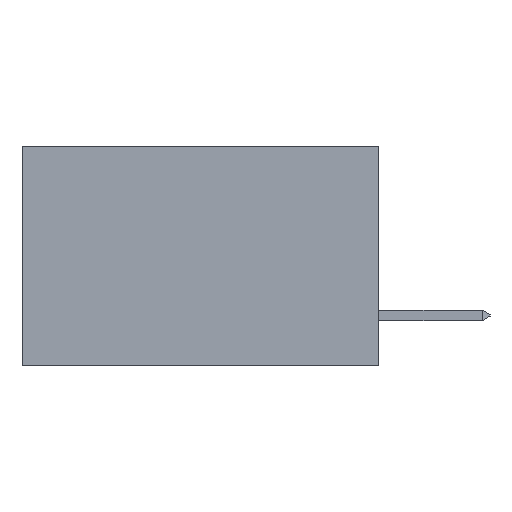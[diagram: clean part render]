
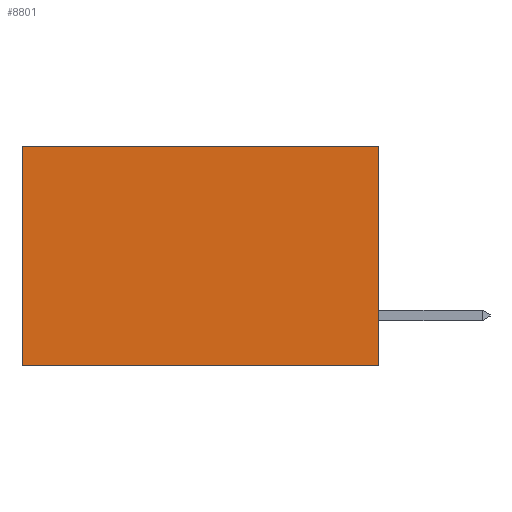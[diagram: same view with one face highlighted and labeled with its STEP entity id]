
A CAD part, left-side view. The second image highlights one B-rep face of the part: STEP entity #8801.
In plain terms, the highlighted planar face has unit normal (-1, 0, 0).
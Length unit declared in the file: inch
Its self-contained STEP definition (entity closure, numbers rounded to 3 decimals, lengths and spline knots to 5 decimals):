
#38 = CARTESIAN_POINT ( 'NONE',  ( 0.298, 0., 0. ) ) ;
#959 = VERTEX_POINT ( 'NONE', #13159 ) ;
#1325 = VERTEX_POINT ( 'NONE', #5089 ) ;
#2622 = EDGE_CURVE ( 'NONE', #1325, #959, #25353, .T. ) ;
#3400 = ORIENTED_EDGE ( 'NONE', *, *, #13935, .T. ) ;
#4937 = VECTOR ( 'NONE', #25091, 39.37008 ) ;
#5089 = CARTESIAN_POINT ( 'NONE',  ( 0.298, 0., 0. ) ) ;
#5560 = LINE ( 'NONE', #11406, #4937 ) ;
#7780 = EDGE_CURVE ( 'NONE', #24467, #10769, #17900, .T. ) ;
#8230 = ORIENTED_EDGE ( 'NONE', *, *, #7780, .T. ) ;
#8351 = ORIENTED_EDGE ( 'NONE', *, *, #12452, .F. ) ;
#8801 = ADVANCED_FACE ( 'NONE', ( #18733 ), #14716, .F. ) ;
#9510 = DIRECTION ( 'NONE',  ( 0., 0., -1. ) ) ;
#9534 = CARTESIAN_POINT ( 'NONE',  ( 0.298, 0.6, 0. ) ) ;
#9561 = LINE ( 'NONE', #10772, #24588 ) ;
#10769 = VERTEX_POINT ( 'NONE', #15566 ) ;
#10772 = CARTESIAN_POINT ( 'NONE',  ( 0.298, 0., 0. ) ) ;
#10871 = DIRECTION ( 'NONE',  ( 0., 0., -1. ) ) ;
#11406 = CARTESIAN_POINT ( 'NONE',  ( 0.298, 0., -0.37 ) ) ;
#11749 = CARTESIAN_POINT ( 'NONE',  ( 0.298, 0.6, 0. ) ) ;
#12336 = DIRECTION ( 'NONE',  ( 1., 0., 0. ) ) ;
#12452 = EDGE_CURVE ( 'NONE', #959, #10769, #5560, .T. ) ;
#12770 = DIRECTION ( 'NONE',  ( 0., 1., 0. ) ) ;
#12783 = CARTESIAN_POINT ( 'NONE',  ( 0.298, 0., 0. ) ) ;
#13034 = DIRECTION ( 'NONE',  ( 0., 0., -1. ) ) ;
#13159 = CARTESIAN_POINT ( 'NONE',  ( 0.298, 0., -0.37 ) ) ;
#13253 = VECTOR ( 'NONE', #9510, 39.37008 ) ;
#13935 = EDGE_CURVE ( 'NONE', #1325, #24467, #9561, .T. ) ;
#14376 = VECTOR ( 'NONE', #13034, 39.37008 ) ;
#14716 = PLANE ( 'NONE',  #15049 ) ;
#15049 = AXIS2_PLACEMENT_3D ( 'NONE', #38, #12336, #10871 ) ;
#15566 = CARTESIAN_POINT ( 'NONE',  ( 0.298, 0.6, -0.37 ) ) ;
#15624 = ORIENTED_EDGE ( 'NONE', *, *, #2622, .F. ) ;
#17858 = EDGE_LOOP ( 'NONE', ( #8230, #8351, #15624, #3400 ) ) ;
#17900 = LINE ( 'NONE', #9534, #13253 ) ;
#18733 = FACE_OUTER_BOUND ( 'NONE', #17858, .T. ) ;
#24467 = VERTEX_POINT ( 'NONE', #11749 ) ;
#24588 = VECTOR ( 'NONE', #12770, 39.37008 ) ;
#25091 = DIRECTION ( 'NONE',  ( 0., 1., 0. ) ) ;
#25353 = LINE ( 'NONE', #12783, #14376 ) ;
